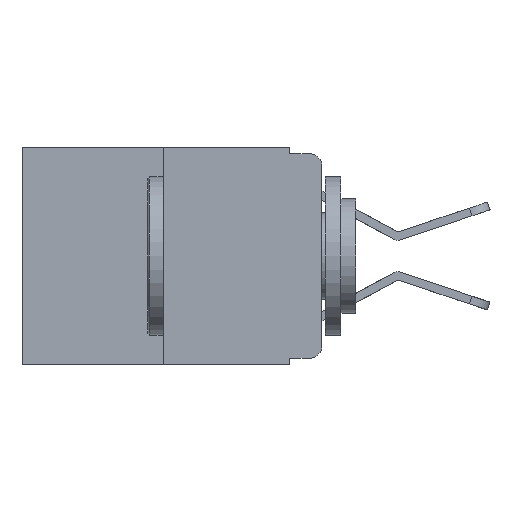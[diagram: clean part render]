
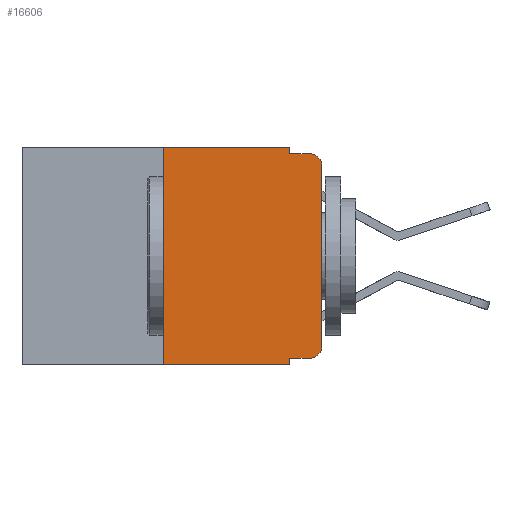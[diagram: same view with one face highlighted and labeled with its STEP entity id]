
A CAD part, left-side view. The second image highlights one B-rep face of the part: STEP entity #16606.
In plain terms, the highlighted planar face has unit normal (-1, 0, 0).
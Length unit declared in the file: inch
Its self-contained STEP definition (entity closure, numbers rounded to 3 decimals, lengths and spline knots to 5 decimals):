
#146 = EDGE_CURVE ( 'NONE', #14192, #13222, #5772, .T. ) ;
#173 = CARTESIAN_POINT ( 'NONE',  ( 0., 0.02, -0.01 ) ) ;
#712 = VERTEX_POINT ( 'NONE', #3399 ) ;
#791 = VECTOR ( 'NONE', #17581, 39.37008 ) ;
#995 = EDGE_CURVE ( 'NONE', #12662, #18988, #9409, .T. ) ;
#1125 = CARTESIAN_POINT ( 'NONE',  ( 0., 0.25, 0. ) ) ;
#1214 = LINE ( 'NONE', #9666, #9091 ) ;
#1220 = CARTESIAN_POINT ( 'NONE',  ( 0., 0.02, -0.03 ) ) ;
#1321 = LINE ( 'NONE', #6316, #12823 ) ;
#2324 = ORIENTED_EDGE ( 'NONE', *, *, #15915, .F. ) ;
#2345 = EDGE_CURVE ( 'NONE', #14192, #19418, #3585, .T. ) ;
#2530 = VECTOR ( 'NONE', #14385, 39.37008 ) ;
#2808 = DIRECTION ( 'NONE',  ( 0., 0., -1. ) ) ;
#2881 = VERTEX_POINT ( 'NONE', #173 ) ;
#3024 = LINE ( 'NONE', #13796, #8189 ) ;
#3109 = DIRECTION ( 'NONE',  ( 0., -1., 0. ) ) ;
#3399 = CARTESIAN_POINT ( 'NONE',  ( 0., 0.051, -0.01 ) ) ;
#3585 = LINE ( 'NONE', #1125, #19529 ) ;
#3750 = AXIS2_PLACEMENT_3D ( 'NONE', #1220, #12172, #2808 ) ;
#3846 = PLANE ( 'NONE',  #8866 ) ;
#4138 = CARTESIAN_POINT ( 'NONE',  ( 0., 0.051, 0. ) ) ;
#4879 = CARTESIAN_POINT ( 'NONE',  ( 0., 0., -0.03 ) ) ;
#5434 = DIRECTION ( 'NONE',  ( 0., 0., -1. ) ) ;
#5772 = LINE ( 'NONE', #10197, #2530 ) ;
#5958 = AXIS2_PLACEMENT_3D ( 'NONE', #9141, #19877, #10712 ) ;
#6175 = EDGE_CURVE ( 'NONE', #19929, #712, #16774, .T. ) ;
#6316 = CARTESIAN_POINT ( 'NONE',  ( 0., 0.051, -0.333 ) ) ;
#6933 = FACE_OUTER_BOUND ( 'NONE', #13897, .T. ) ;
#7431 = CARTESIAN_POINT ( 'NONE',  ( 0., 0.25, 0. ) ) ;
#7695 = LINE ( 'NONE', #8357, #791 ) ;
#7716 = CIRCLE ( 'NONE', #3750, 0.02 ) ;
#7959 = CARTESIAN_POINT ( 'NONE',  ( 0., 0.02, -0.333 ) ) ;
#8189 = VECTOR ( 'NONE', #18327, 39.37008 ) ;
#8357 = CARTESIAN_POINT ( 'NONE',  ( 0., 0.051, 0. ) ) ;
#8433 = ORIENTED_EDGE ( 'NONE', *, *, #15519, .T. ) ;
#8866 = AXIS2_PLACEMENT_3D ( 'NONE', #10049, #14704, #5434 ) ;
#8931 = VECTOR ( 'NONE', #10158, 39.37008 ) ;
#8970 = ORIENTED_EDGE ( 'NONE', *, *, #10455, .F. ) ;
#9091 = VECTOR ( 'NONE', #15859, 39.37008 ) ;
#9141 = CARTESIAN_POINT ( 'NONE',  ( 0., 0.02, -0.313 ) ) ;
#9200 = ORIENTED_EDGE ( 'NONE', *, *, #6175, .F. ) ;
#9205 = CARTESIAN_POINT ( 'NONE',  ( 0., 0.051, -0.343 ) ) ;
#9409 = LINE ( 'NONE', #10988, #8931 ) ;
#9499 = CARTESIAN_POINT ( 'NONE',  ( 0., 0., -0.313 ) ) ;
#9666 = CARTESIAN_POINT ( 'NONE',  ( 0., 0.051, -0.01 ) ) ;
#9859 = EDGE_CURVE ( 'NONE', #10637, #20082, #1321, .T. ) ;
#10049 = CARTESIAN_POINT ( 'NONE',  ( 0., 0.473, 0. ) ) ;
#10158 = DIRECTION ( 'NONE',  ( 0., 0., 1. ) ) ;
#10197 = CARTESIAN_POINT ( 'NONE',  ( 0., 0.473, -0.343 ) ) ;
#10322 = CIRCLE ( 'NONE', #5958, 0.02 ) ;
#10455 = EDGE_CURVE ( 'NONE', #19418, #19929, #3024, .T. ) ;
#10637 = VERTEX_POINT ( 'NONE', #19128 ) ;
#10712 = DIRECTION ( 'NONE',  ( 0., 0., -1. ) ) ;
#10988 = CARTESIAN_POINT ( 'NONE',  ( 0., 0., 0. ) ) ;
#11418 = ORIENTED_EDGE ( 'NONE', *, *, #2345, .F. ) ;
#12172 = DIRECTION ( 'NONE',  ( -1., 0., 0. ) ) ;
#12185 = EDGE_CURVE ( 'NONE', #20082, #12662, #10322, .T. ) ;
#12589 = ORIENTED_EDGE ( 'NONE', *, *, #9859, .T. ) ;
#12662 = VERTEX_POINT ( 'NONE', #9499 ) ;
#12823 = VECTOR ( 'NONE', #3109, 39.37008 ) ;
#13222 = VERTEX_POINT ( 'NONE', #9205 ) ;
#13337 = CARTESIAN_POINT ( 'NONE',  ( 0., 0.051, 0. ) ) ;
#13414 = CARTESIAN_POINT ( 'NONE',  ( 0., 0.25, -0.343 ) ) ;
#13796 = CARTESIAN_POINT ( 'NONE',  ( 0., 0.473, 0. ) ) ;
#13897 = EDGE_LOOP ( 'NONE', ( #14231, #8433, #19024, #9200, #8970, #11418, #15961, #2324, #12589, #19052 ) ) ;
#14192 = VERTEX_POINT ( 'NONE', #13414 ) ;
#14231 = ORIENTED_EDGE ( 'NONE', *, *, #995, .T. ) ;
#14385 = DIRECTION ( 'NONE',  ( 0., -1., 0. ) ) ;
#14704 = DIRECTION ( 'NONE',  ( 1., 0., 0. ) ) ;
#15519 = EDGE_CURVE ( 'NONE', #18988, #2881, #7716, .T. ) ;
#15859 = DIRECTION ( 'NONE',  ( 0., -1., 0. ) ) ;
#15915 = EDGE_CURVE ( 'NONE', #10637, #13222, #7695, .T. ) ;
#15961 = ORIENTED_EDGE ( 'NONE', *, *, #146, .T. ) ;
#16308 = VECTOR ( 'NONE', #16433, 39.37008 ) ;
#16433 = DIRECTION ( 'NONE',  ( 0., 0., -1. ) ) ;
#16606 = ADVANCED_FACE ( 'NONE', ( #6933 ), #3846, .F. ) ;
#16774 = LINE ( 'NONE', #13337, #16308 ) ;
#17581 = DIRECTION ( 'NONE',  ( 0., 0., -1. ) ) ;
#18177 = EDGE_CURVE ( 'NONE', #712, #2881, #1214, .T. ) ;
#18327 = DIRECTION ( 'NONE',  ( 0., -1., 0. ) ) ;
#18904 = DIRECTION ( 'NONE',  ( 0., 0., 1. ) ) ;
#18988 = VERTEX_POINT ( 'NONE', #4879 ) ;
#19024 = ORIENTED_EDGE ( 'NONE', *, *, #18177, .F. ) ;
#19052 = ORIENTED_EDGE ( 'NONE', *, *, #12185, .T. ) ;
#19128 = CARTESIAN_POINT ( 'NONE',  ( 0., 0.051, -0.333 ) ) ;
#19418 = VERTEX_POINT ( 'NONE', #7431 ) ;
#19529 = VECTOR ( 'NONE', #18904, 39.37008 ) ;
#19877 = DIRECTION ( 'NONE',  ( -1., 0., 0. ) ) ;
#19929 = VERTEX_POINT ( 'NONE', #4138 ) ;
#20082 = VERTEX_POINT ( 'NONE', #7959 ) ;
